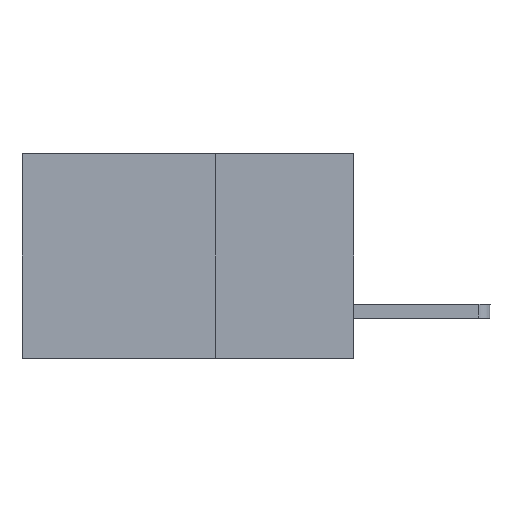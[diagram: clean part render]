
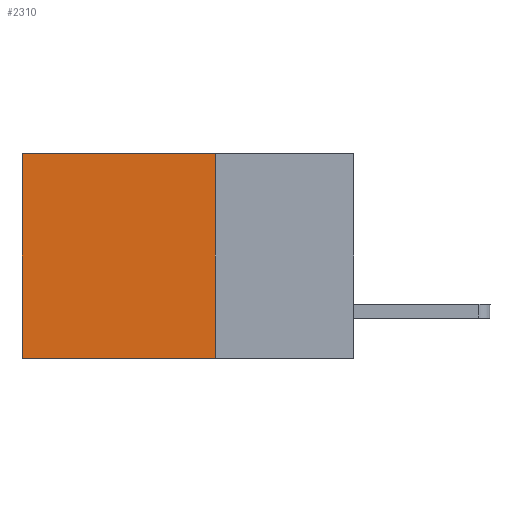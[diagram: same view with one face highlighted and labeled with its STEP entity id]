
A CAD part, left-side view. The second image highlights one B-rep face of the part: STEP entity #2310.
In plain terms, the highlighted planar face has unit normal (-1, 0, 0).
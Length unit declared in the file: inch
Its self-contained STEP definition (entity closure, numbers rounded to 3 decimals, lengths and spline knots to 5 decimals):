
#47 = EDGE_CURVE ( 'NONE', #2746, #1459, #7631, .T. ) ;
#150 = EDGE_CURVE ( 'NONE', #2309, #1459, #6579, .T. ) ;
#216 = DIRECTION ( 'NONE',  ( 0., 1., 0. ) ) ;
#955 = VECTOR ( 'NONE', #8337, 39.37008 ) ;
#1144 = ORIENTED_EDGE ( 'NONE', *, *, #150, .T. ) ;
#1459 = VERTEX_POINT ( 'NONE', #6048 ) ;
#1806 = ORIENTED_EDGE ( 'NONE', *, *, #3682, .F. ) ;
#2309 = VERTEX_POINT ( 'NONE', #7280 ) ;
#2310 = ADVANCED_FACE ( 'NONE', ( #6207 ), #2605, .F. ) ;
#2601 = VECTOR ( 'NONE', #7890, 39.37008 ) ;
#2605 = PLANE ( 'NONE',  #8455 ) ;
#2721 = CARTESIAN_POINT ( 'NONE',  ( 0.2875, 0.25, 0. ) ) ;
#2746 = VERTEX_POINT ( 'NONE', #5768 ) ;
#2931 = ORIENTED_EDGE ( 'NONE', *, *, #47, .F. ) ;
#3004 = EDGE_CURVE ( 'NONE', #5246, #2309, #7315, .T. ) ;
#3682 = EDGE_CURVE ( 'NONE', #5246, #2746, #6283, .T. ) ;
#3849 = CARTESIAN_POINT ( 'NONE',  ( 0.2875, 0.6, 0. ) ) ;
#4259 = VECTOR ( 'NONE', #7235, 39.37008 ) ;
#4540 = CARTESIAN_POINT ( 'NONE',  ( 0.2875, 0.25, 0. ) ) ;
#4555 = DIRECTION ( 'NONE',  ( 1., 0., 0. ) ) ;
#4583 = DIRECTION ( 'NONE',  ( 0., 0., -1. ) ) ;
#5246 = VERTEX_POINT ( 'NONE', #2721 ) ;
#5768 = CARTESIAN_POINT ( 'NONE',  ( 0.2875, 0.25, -0.37 ) ) ;
#6048 = CARTESIAN_POINT ( 'NONE',  ( 0.2875, 0.6, -0.37 ) ) ;
#6207 = FACE_OUTER_BOUND ( 'NONE', #6322, .T. ) ;
#6283 = LINE ( 'NONE', #8430, #955 ) ;
#6322 = EDGE_LOOP ( 'NONE', ( #1144, #2931, #1806, #8588 ) ) ;
#6579 = LINE ( 'NONE', #3849, #2601 ) ;
#6884 = CARTESIAN_POINT ( 'NONE',  ( 0.2875, 0.25, -0.37 ) ) ;
#7235 = DIRECTION ( 'NONE',  ( 0., 1., 0. ) ) ;
#7280 = CARTESIAN_POINT ( 'NONE',  ( 0.2875, 0.6, 0. ) ) ;
#7315 = LINE ( 'NONE', #4540, #4259 ) ;
#7426 = VECTOR ( 'NONE', #216, 39.37008 ) ;
#7631 = LINE ( 'NONE', #6884, #7426 ) ;
#7890 = DIRECTION ( 'NONE',  ( 0., 0., -1. ) ) ;
#7957 = CARTESIAN_POINT ( 'NONE',  ( 0.2875, 0.25, 0. ) ) ;
#8337 = DIRECTION ( 'NONE',  ( 0., 0., -1. ) ) ;
#8430 = CARTESIAN_POINT ( 'NONE',  ( 0.2875, 0.25, 0. ) ) ;
#8455 = AXIS2_PLACEMENT_3D ( 'NONE', #7957, #4555, #4583 ) ;
#8588 = ORIENTED_EDGE ( 'NONE', *, *, #3004, .T. ) ;
